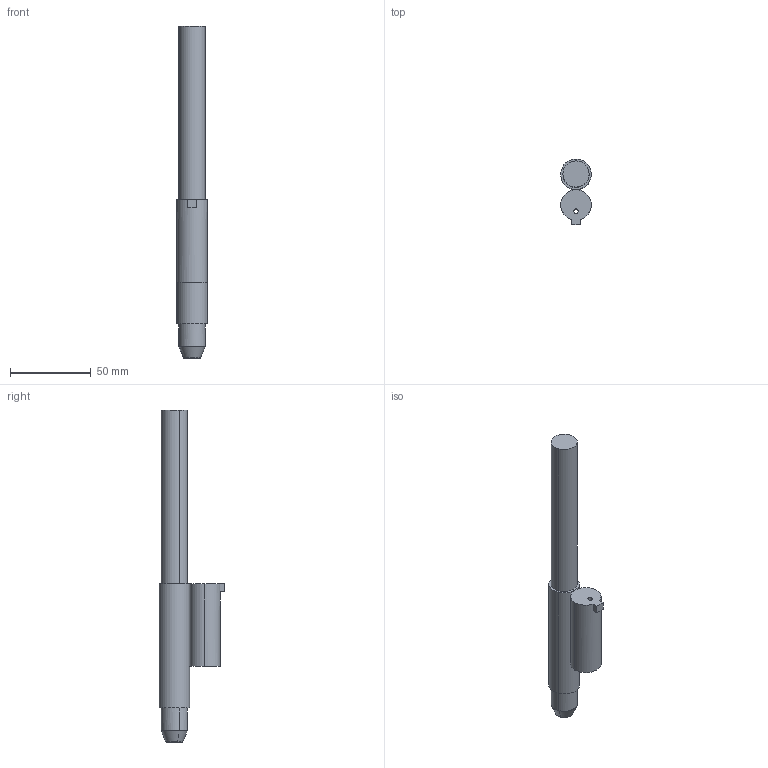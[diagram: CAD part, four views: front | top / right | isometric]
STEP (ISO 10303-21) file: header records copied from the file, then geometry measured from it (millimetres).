
FILE_DESCRIPTION (( 'STEP AP203' ), '1' );
FILE_NAME ('bolt assy.STEP', '2020-09-09T05:34:52', ( '' ), ( '' ), 'SwSTEP 2.0', 'SolidWorks 2019', '' );
FILE_SCHEMA (( 'CONFIG_CONTROL_DESIGN' ));
Length unit declared in the file: millimetre
Products named in the file (3): lower bolt; upper bolt.stp; bolt assy
Assembly tree (2 placements, depth 2):
  bolt assy
    lower bolt
    upper bolt.stp
Bounding box: 19 x 40.96 x 206.2 mm (x, y, z)
Volume: 62479.7 mm3; surface area: 15814.1 mm2
Topology: 2 solids, 2 shells, 29 faces, 60 edges, 38 vertices
Faces by surface type: cylinder 12, plane 11, cone 4, bspline 2
Entity records: 1365 total; most frequent: CARTESIAN_POINT 432, DIRECTION 146, ORIENTED_EDGE 120, EDGE_CURVE 60, AXIS2_PLACEMENT_3D 60, VERTEX_POINT 38, EDGE_LOOP 34, ADVANCED_FACE 29
